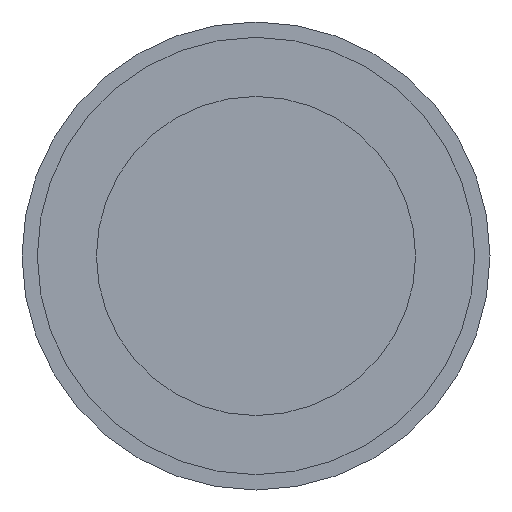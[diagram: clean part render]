
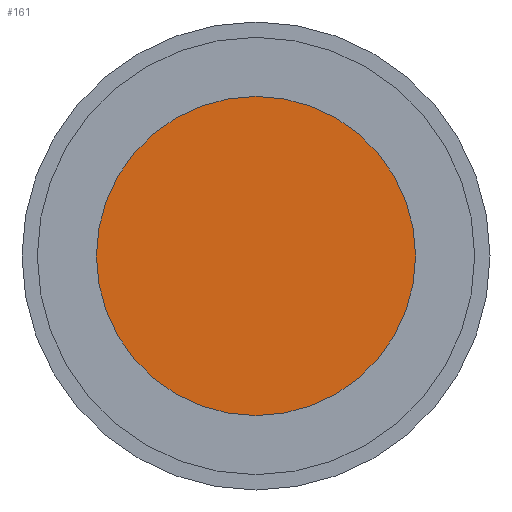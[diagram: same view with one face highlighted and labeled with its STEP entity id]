
A CAD part, front view. The second image highlights one B-rep face of the part: STEP entity #161.
In plain terms, the highlighted planar face has unit normal (0, -1, 0).
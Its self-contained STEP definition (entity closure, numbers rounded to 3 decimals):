
#69 = VERTEX_POINT ( 'NONE', #93 ) ;
#77 = CIRCLE ( 'NONE', #117, 6.75 ) ;
#82 = FACE_OUTER_BOUND ( 'NONE', #129, .T. ) ;
#93 = CARTESIAN_POINT ( 'NONE',  ( 0., 30., -6.75 ) ) ;
#114 = DIRECTION ( 'NONE',  ( 0., -1., 0. ) ) ;
#117 = AXIS2_PLACEMENT_3D ( 'NONE', #131, #138, #135 ) ;
#120 = AXIS2_PLACEMENT_3D ( 'NONE', #173, #114, #166 ) ;
#129 = EDGE_LOOP ( 'NONE', ( #134 ) ) ;
#131 = CARTESIAN_POINT ( 'NONE',  ( 0., 30., 0. ) ) ;
#134 = ORIENTED_EDGE ( 'NONE', *, *, #164, .T. ) ;
#135 = DIRECTION ( 'NONE',  ( 0., 0., -1. ) ) ;
#138 = DIRECTION ( 'NONE',  ( 0., -1., 0. ) ) ;
#161 = ADVANCED_FACE ( 'NONE', ( #82 ), #171, .T. ) ;
#164 = EDGE_CURVE ( 'NONE', #69, #69, #77, .T. ) ;
#166 = DIRECTION ( 'NONE',  ( 0., 0., -1. ) ) ;
#171 = PLANE ( 'NONE',  #120 ) ;
#173 = CARTESIAN_POINT ( 'NONE',  ( 0., 30., 0. ) ) ;
